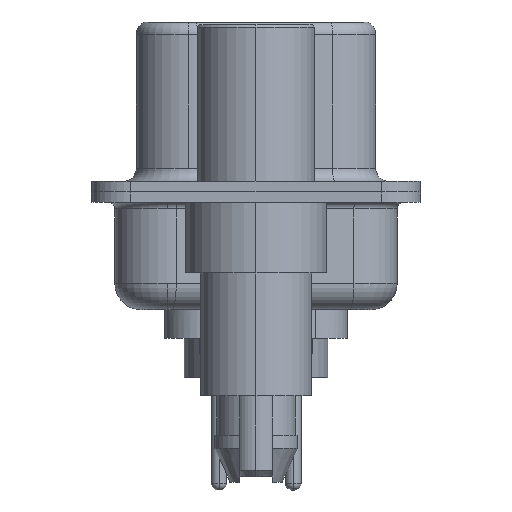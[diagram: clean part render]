
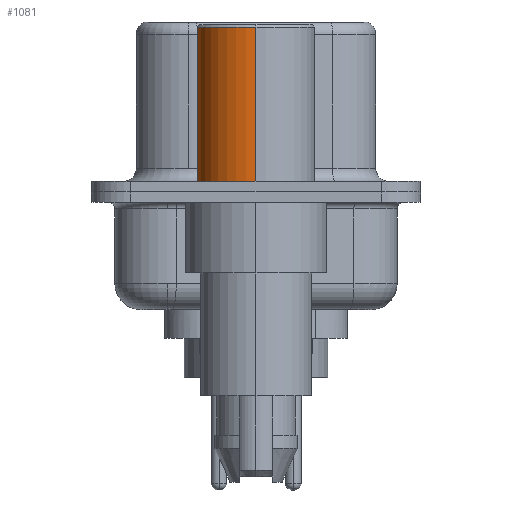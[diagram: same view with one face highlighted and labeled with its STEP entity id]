
A CAD part, left-side view. The second image highlights one B-rep face of the part: STEP entity #1081.
In plain terms, the highlighted cylindrical face has radius 2.25 mm (diameter 4.5 mm), a partial arc.
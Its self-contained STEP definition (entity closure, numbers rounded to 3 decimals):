
#1081 = ADVANCED_FACE ( 'NONE', ( #6100 ), #12800, .T. ) ;
#1246 = DIRECTION ( 'NONE',  ( 0., 0., 1. ) ) ;
#2175 = CARTESIAN_POINT ( 'NONE',  ( 2.25, 0., 6.3 ) ) ;
#2536 = VERTEX_POINT ( 'NONE', #9363 ) ;
#2778 = DIRECTION ( 'NONE',  ( 1., 0., 0. ) ) ;
#2789 = ORIENTED_EDGE ( 'NONE', *, *, #5352, .F. ) ;
#2868 = VERTEX_POINT ( 'NONE', #13120 ) ;
#2924 = DIRECTION ( 'NONE',  ( 0., 0., 1. ) ) ;
#2936 = DIRECTION ( 'NONE',  ( 1., 0., 0. ) ) ;
#3510 = CARTESIAN_POINT ( 'NONE',  ( 2.25, 0., 0.581 ) ) ;
#3554 = EDGE_CURVE ( 'NONE', #2868, #8076, #14015, .T. ) ;
#3668 = VECTOR ( 'NONE', #5250, 1000. ) ;
#3862 = EDGE_CURVE ( 'NONE', #2868, #4993, #6655, .T. ) ;
#4688 = AXIS2_PLACEMENT_3D ( 'NONE', #14732, #8333, #14917 ) ;
#4993 = VERTEX_POINT ( 'NONE', #8488 ) ;
#5250 = DIRECTION ( 'NONE',  ( 0., 0., 1. ) ) ;
#5352 = EDGE_CURVE ( 'NONE', #8076, #2536, #7465, .T. ) ;
#5537 = LINE ( 'NONE', #9667, #8266 ) ;
#5871 = EDGE_LOOP ( 'NONE', ( #15273, #10653, #2789, #10306 ) ) ;
#6100 = FACE_OUTER_BOUND ( 'NONE', #5871, .T. ) ;
#6655 = CIRCLE ( 'NONE', #9120, 2.25 ) ;
#7465 = CIRCLE ( 'NONE', #11076, 2.25 ) ;
#8076 = VERTEX_POINT ( 'NONE', #2175 ) ;
#8266 = VECTOR ( 'NONE', #8361, 1000. ) ;
#8333 = DIRECTION ( 'NONE',  ( 0., 0., 1. ) ) ;
#8361 = DIRECTION ( 'NONE',  ( 0., 0., 1. ) ) ;
#8488 = CARTESIAN_POINT ( 'NONE',  ( -2.25, 0., 0.4 ) ) ;
#9120 = AXIS2_PLACEMENT_3D ( 'NONE', #11252, #2924, #2936 ) ;
#9363 = CARTESIAN_POINT ( 'NONE',  ( -2.25, 0., 6.3 ) ) ;
#9667 = CARTESIAN_POINT ( 'NONE',  ( -2.25, 0., 0.581 ) ) ;
#10306 = ORIENTED_EDGE ( 'NONE', *, *, #3554, .F. ) ;
#10653 = ORIENTED_EDGE ( 'NONE', *, *, #17297, .T. ) ;
#11076 = AXIS2_PLACEMENT_3D ( 'NONE', #16871, #1246, #2778 ) ;
#11252 = CARTESIAN_POINT ( 'NONE',  ( 0., 0., 0.4 ) ) ;
#12800 = CYLINDRICAL_SURFACE ( 'NONE', #4688, 2.25 ) ;
#13120 = CARTESIAN_POINT ( 'NONE',  ( 2.25, 0., 0.4 ) ) ;
#14015 = LINE ( 'NONE', #3510, #3668 ) ;
#14732 = CARTESIAN_POINT ( 'NONE',  ( 0., 0., 0.581 ) ) ;
#14917 = DIRECTION ( 'NONE',  ( 1., 0., 0. ) ) ;
#15273 = ORIENTED_EDGE ( 'NONE', *, *, #3862, .T. ) ;
#16871 = CARTESIAN_POINT ( 'NONE',  ( 0., 0., 6.3 ) ) ;
#17297 = EDGE_CURVE ( 'NONE', #4993, #2536, #5537, .T. ) ;
